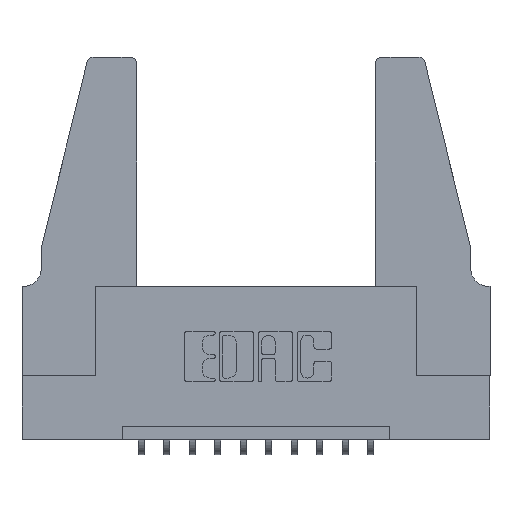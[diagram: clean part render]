
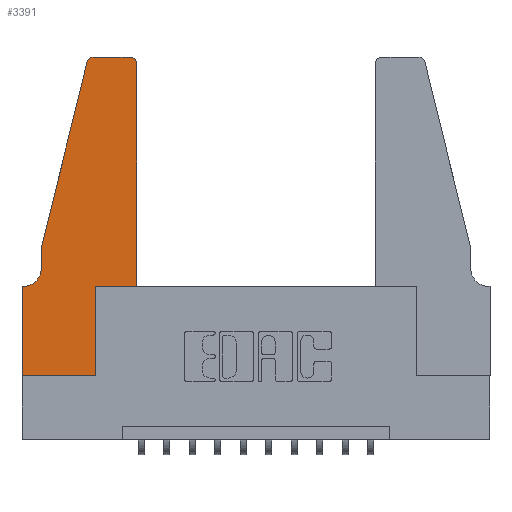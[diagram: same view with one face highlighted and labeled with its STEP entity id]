
A CAD part, top view. The second image highlights one B-rep face of the part: STEP entity #3391.
In plain terms, the highlighted planar face has unit normal (0, 0, 1).
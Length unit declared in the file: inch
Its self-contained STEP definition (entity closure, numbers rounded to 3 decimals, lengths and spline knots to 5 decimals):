
#84 = DIRECTION ( 'NONE',  ( 0., 0., 1. ) ) ;
#94 = LINE ( 'NONE', #6009, #10239 ) ;
#159 = VECTOR ( 'NONE', #3080, 39.37008 ) ;
#489 = ORIENTED_EDGE ( 'NONE', *, *, #6275, .T. ) ;
#614 = DIRECTION ( 'NONE',  ( 0., 0., -1. ) ) ;
#624 = LINE ( 'NONE', #9111, #2993 ) ;
#629 = EDGE_CURVE ( 'NONE', #2112, #3297, #624, .T. ) ;
#658 = AXIS2_PLACEMENT_3D ( 'NONE', #14065, #84, #12053 ) ;
#674 = CARTESIAN_POINT ( 'NONE',  ( 0., 0., 0.37 ) ) ;
#755 = EDGE_CURVE ( 'NONE', #11014, #9231, #10093, .T. ) ;
#923 = EDGE_CURVE ( 'NONE', #3297, #5374, #3863, .T. ) ;
#976 = VECTOR ( 'NONE', #10306, 39.37008 ) ;
#1068 = VERTEX_POINT ( 'NONE', #8036 ) ;
#1499 = DIRECTION ( 'NONE',  ( 0., 0., 1. ) ) ;
#1680 = DIRECTION ( 'NONE',  ( -1., 0., 0. ) ) ;
#1707 = EDGE_CURVE ( 'NONE', #13242, #4422, #13170, .T. ) ;
#1826 = CARTESIAN_POINT ( 'NONE',  ( 0.0755, 0.5, 0.37 ) ) ;
#2026 = CARTESIAN_POINT ( 'NONE',  ( 0.2605, 1.25, 0.37 ) ) ;
#2112 = VERTEX_POINT ( 'NONE', #1826 ) ;
#2381 = LINE ( 'NONE', #9748, #5784 ) ;
#2723 = LINE ( 'NONE', #2026, #159 ) ;
#2816 = DIRECTION ( 'NONE',  ( 0., -1., 0. ) ) ;
#2993 = VECTOR ( 'NONE', #6922, 39.37008 ) ;
#3076 = VECTOR ( 'NONE', #13228, 39.37008 ) ;
#3080 = DIRECTION ( 'NONE',  ( -1., 0., 0. ) ) ;
#3260 = DIRECTION ( 'NONE',  ( 1., 0., 0. ) ) ;
#3275 = CARTESIAN_POINT ( 'NONE',  ( 0.4205, 1.22, 0.37 ) ) ;
#3297 = VERTEX_POINT ( 'NONE', #4078 ) ;
#3391 = ADVANCED_FACE ( 'NONE', ( #6322 ), #6452, .T. ) ;
#3459 = EDGE_CURVE ( 'NONE', #5374, #13715, #13791, .T. ) ;
#3510 = CARTESIAN_POINT ( 'NONE',  ( 0.4505, 1.22, 0.37 ) ) ;
#3528 = CARTESIAN_POINT ( 'NONE',  ( 0.4205, 1.25, 0.37 ) ) ;
#3571 = CARTESIAN_POINT ( 'NONE',  ( 0.2865, 0.35, 0.37 ) ) ;
#3649 = CARTESIAN_POINT ( 'NONE',  ( 0.0755, 0.35, 0.37 ) ) ;
#3863 = CIRCLE ( 'NONE', #7626, 0.07 ) ;
#3971 = ORIENTED_EDGE ( 'NONE', *, *, #10084, .T. ) ;
#4078 = CARTESIAN_POINT ( 'NONE',  ( 0.0755, 0.42, 0.37 ) ) ;
#4183 = CARTESIAN_POINT ( 'NONE',  ( 0., 0., 0.37 ) ) ;
#4422 = VERTEX_POINT ( 'NONE', #3528 ) ;
#4561 = CARTESIAN_POINT ( 'NONE',  ( 0.4505, 0.35, 0.37 ) ) ;
#4713 = LINE ( 'NONE', #11278, #976 ) ;
#5185 = ORIENTED_EDGE ( 'NONE', *, *, #3459, .T. ) ;
#5227 = EDGE_CURVE ( 'NONE', #4422, #1068, #2723, .T. ) ;
#5270 = EDGE_CURVE ( 'NONE', #9231, #9848, #2381, .T. ) ;
#5277 = AXIS2_PLACEMENT_3D ( 'NONE', #3275, #10862, #5943 ) ;
#5341 = CARTESIAN_POINT ( 'NONE',  ( 0., 0.35, 0.37 ) ) ;
#5374 = VERTEX_POINT ( 'NONE', #11225 ) ;
#5417 = CARTESIAN_POINT ( 'NONE',  ( 0.2865, 0., 0.37 ) ) ;
#5619 = CARTESIAN_POINT ( 'NONE',  ( 0.2865, 0.35, 0.37 ) ) ;
#5784 = VECTOR ( 'NONE', #8610, 39.37008 ) ;
#5788 = ORIENTED_EDGE ( 'NONE', *, *, #923, .T. ) ;
#5821 = VERTEX_POINT ( 'NONE', #674 ) ;
#5943 = DIRECTION ( 'NONE',  ( 1., 0., 0. ) ) ;
#5950 = CARTESIAN_POINT ( 'NONE',  ( 0.284, 1.22, 0.37 ) ) ;
#5986 = CARTESIAN_POINT ( 'NONE',  ( 0.0055, 0.42, 0.37 ) ) ;
#6009 = CARTESIAN_POINT ( 'NONE',  ( 0., 0., 0.37 ) ) ;
#6275 = EDGE_CURVE ( 'NONE', #1068, #6749, #12253, .T. ) ;
#6322 = FACE_OUTER_BOUND ( 'NONE', #8564, .T. ) ;
#6450 = ORIENTED_EDGE ( 'NONE', *, *, #10231, .T. ) ;
#6452 = PLANE ( 'NONE',  #658 ) ;
#6557 = LINE ( 'NONE', #8364, #7223 ) ;
#6593 = ORIENTED_EDGE ( 'NONE', *, *, #13534, .T. ) ;
#6749 = VERTEX_POINT ( 'NONE', #11891 ) ;
#6922 = DIRECTION ( 'NONE',  ( 0., -1., 0. ) ) ;
#7146 = ORIENTED_EDGE ( 'NONE', *, *, #629, .T. ) ;
#7223 = VECTOR ( 'NONE', #7247, 39.37008 ) ;
#7247 = DIRECTION ( 'NONE',  ( 0., 1., 0. ) ) ;
#7603 = ORIENTED_EDGE ( 'NONE', *, *, #5227, .T. ) ;
#7626 = AXIS2_PLACEMENT_3D ( 'NONE', #5986, #614, #1680 ) ;
#7738 = VECTOR ( 'NONE', #9442, 39.37008 ) ;
#8036 = CARTESIAN_POINT ( 'NONE',  ( 0.284, 1.25, 0.37 ) ) ;
#8364 = CARTESIAN_POINT ( 'NONE',  ( 0.4505, 0.35, 0.37 ) ) ;
#8564 = EDGE_LOOP ( 'NONE', ( #7603, #489, #13983, #7146, #5788, #5185, #6593, #6450, #11115, #12088, #3971, #9767 ) ) ;
#8610 = DIRECTION ( 'NONE',  ( 1., 0., 0. ) ) ;
#8912 = AXIS2_PLACEMENT_3D ( 'NONE', #5950, #1499, #9033 ) ;
#9033 = DIRECTION ( 'NONE',  ( 1., 0., 0. ) ) ;
#9111 = CARTESIAN_POINT ( 'NONE',  ( 0.0755, 0.5, 0.37 ) ) ;
#9231 = VERTEX_POINT ( 'NONE', #5619 ) ;
#9442 = DIRECTION ( 'NONE',  ( 0., 1., 0. ) ) ;
#9748 = CARTESIAN_POINT ( 'NONE',  ( 0.4505, 0.35, 0.37 ) ) ;
#9767 = ORIENTED_EDGE ( 'NONE', *, *, #1707, .T. ) ;
#9848 = VERTEX_POINT ( 'NONE', #4561 ) ;
#10084 = EDGE_CURVE ( 'NONE', #9848, #13242, #6557, .T. ) ;
#10093 = LINE ( 'NONE', #3571, #7738 ) ;
#10231 = EDGE_CURVE ( 'NONE', #5821, #11014, #11292, .T. ) ;
#10239 = VECTOR ( 'NONE', #2816, 39.37008 ) ;
#10241 = VECTOR ( 'NONE', #3260, 39.37008 ) ;
#10306 = DIRECTION ( 'NONE',  ( -0.239, -0.971, 0. ) ) ;
#10862 = DIRECTION ( 'NONE',  ( 0., 0., 1. ) ) ;
#11014 = VERTEX_POINT ( 'NONE', #5417 ) ;
#11115 = ORIENTED_EDGE ( 'NONE', *, *, #755, .T. ) ;
#11225 = CARTESIAN_POINT ( 'NONE',  ( 0.0055, 0.35, 0.37 ) ) ;
#11278 = CARTESIAN_POINT ( 'NONE',  ( 0.0755, 0.5, 0.37 ) ) ;
#11292 = LINE ( 'NONE', #4183, #10241 ) ;
#11891 = CARTESIAN_POINT ( 'NONE',  ( 0.25487, 1.22718, 0.37 ) ) ;
#12053 = DIRECTION ( 'NONE',  ( 1., 0., 0. ) ) ;
#12088 = ORIENTED_EDGE ( 'NONE', *, *, #5270, .T. ) ;
#12253 = CIRCLE ( 'NONE', #8912, 0.03 ) ;
#12890 = EDGE_CURVE ( 'NONE', #6749, #2112, #4713, .T. ) ;
#13170 = CIRCLE ( 'NONE', #5277, 0.03 ) ;
#13228 = DIRECTION ( 'NONE',  ( -1., 0., 0. ) ) ;
#13242 = VERTEX_POINT ( 'NONE', #3510 ) ;
#13534 = EDGE_CURVE ( 'NONE', #13715, #5821, #94, .T. ) ;
#13715 = VERTEX_POINT ( 'NONE', #5341 ) ;
#13791 = LINE ( 'NONE', #3649, #3076 ) ;
#13983 = ORIENTED_EDGE ( 'NONE', *, *, #12890, .T. ) ;
#14065 = CARTESIAN_POINT ( 'NONE',  ( 0., 0.35, 0.37 ) ) ;
